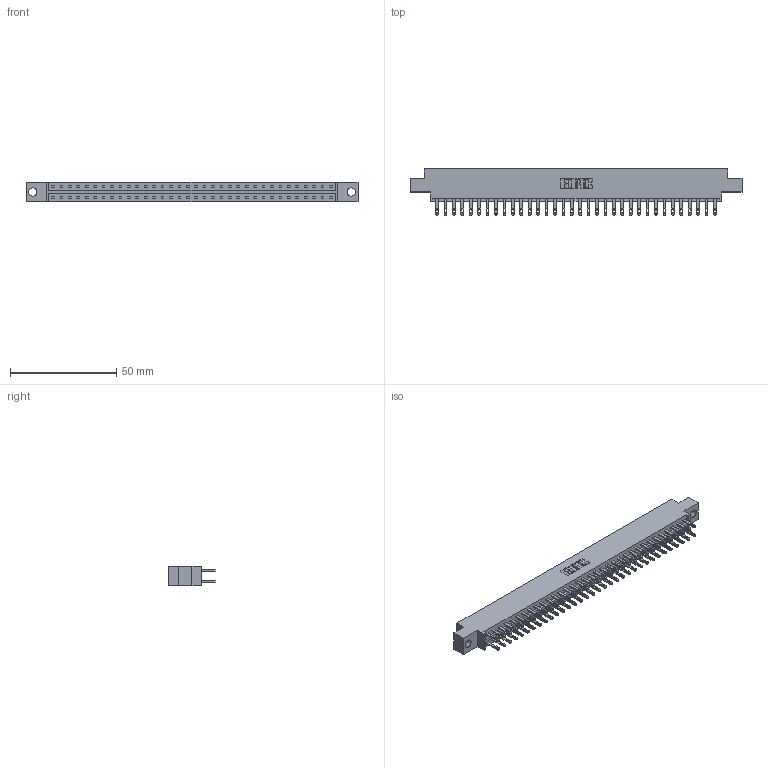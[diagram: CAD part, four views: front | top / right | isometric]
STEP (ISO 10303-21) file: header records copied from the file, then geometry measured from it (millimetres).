
FILE_DESCRIPTION (( 'STEP AP203' ), '1' );
FILE_NAME ('333-068-500-804.STEP', '2018-08-04T12:24:31', ( '' ), ( '' ), 'SwSTEP 2.0', 'SolidWorks 2016', '' );
FILE_SCHEMA (( 'CONFIG_CONTROL_DESIGN' ));
Length unit declared in the file: inch
Products named in the file (3): 333 Part_Offset - .156 Dia - TH; 345-292-001_345-293-100; 333-068-500-804
Assembly tree (69 placements, depth 2):
  333-068-500-804
    333 Part_Offset - .156 Dia - TH
    345-292-001_345-293-100  x68
Bounding box: 156.26 x 21.85 x 9.4 mm (x, y, z)
Volume: 15770.7 mm3; surface area: 19327.4 mm2
Topology: 69 solids, 69 shells, 3382 faces, 10319 edges, 6878 vertices
Faces by surface type: plane 2114, cylinder 1268
Entity records: 22973 total; most frequent: CARTESIAN_POINT 3818, ORIENTED_EDGE 3754, DIRECTION 3277, EDGE_CURVE 1877, LINE 1745, VECTOR 1745, VERTEX_POINT 1250, AXIS2_PLACEMENT_3D 766
